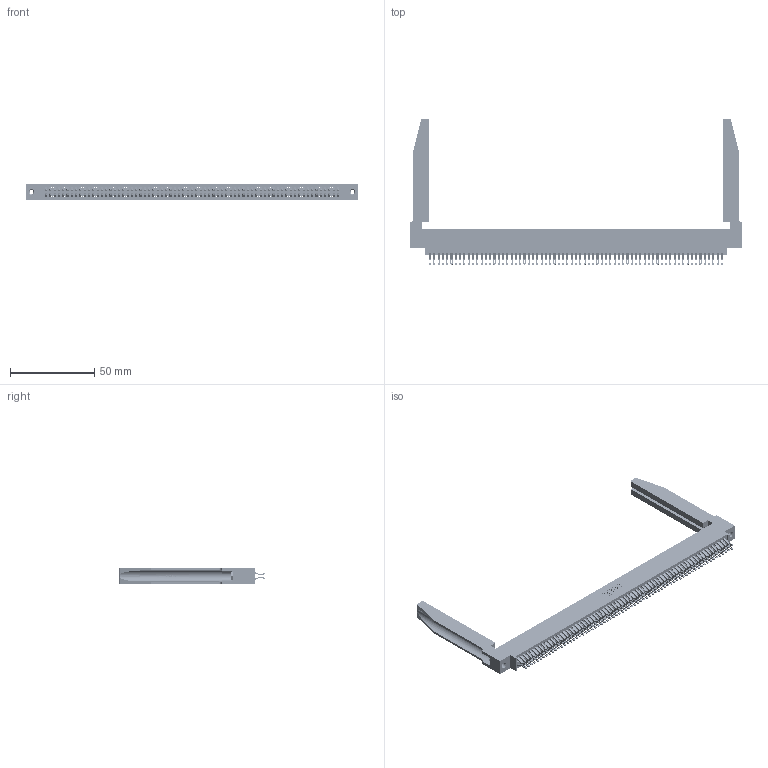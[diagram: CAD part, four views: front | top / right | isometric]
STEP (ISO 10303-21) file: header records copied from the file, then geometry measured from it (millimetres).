
FILE_DESCRIPTION (( 'STEP AP203' ), '1' );
FILE_NAME ('395-138-555-878.STEP', '2019-10-29T21:56:57', ( '' ), ( '' ), 'SwSTEP 2.0', 'SolidWorks 2016', '' );
FILE_SCHEMA (( 'CONFIG_CONTROL_DESIGN' ));
Length unit declared in the file: inch
Products named in the file (5): 345-292-001_555 Tail; 345-250-001_345-250-001-102; 345-220-078_345-220-078; 395-138-555-878; 345 Part_0.170 Offset - 0.156 Dia-TH
Assembly tree (143 placements, depth 2):
  395-138-555-878
    345 Part_0.170 Offset - 0.156 Dia-TH
    345-292-001_555 Tail  x138
    345-250-001_345-250-001-102  x2
    345-220-078_345-220-078  x2
Bounding box: 196.49 x 86.41 x 9.4 mm (x, y, z)
Volume: 27395.6 mm3; surface area: 37906.4 mm2
Topology: 143 solids, 143 shells, 8092 faces, 25387 edges, 16914 vertices
Faces by surface type: plane 4504, cylinder 3536, bspline 36, cone 12, torus 4
Entity records: 55702 total; most frequent: CARTESIAN_POINT 10265, ORIENTED_EDGE 9066, DIRECTION 7979, EDGE_CURVE 4533, VECTOR 4011, LINE 4011, VERTEX_POINT 3016, AXIS2_PLACEMENT_3D 1984
